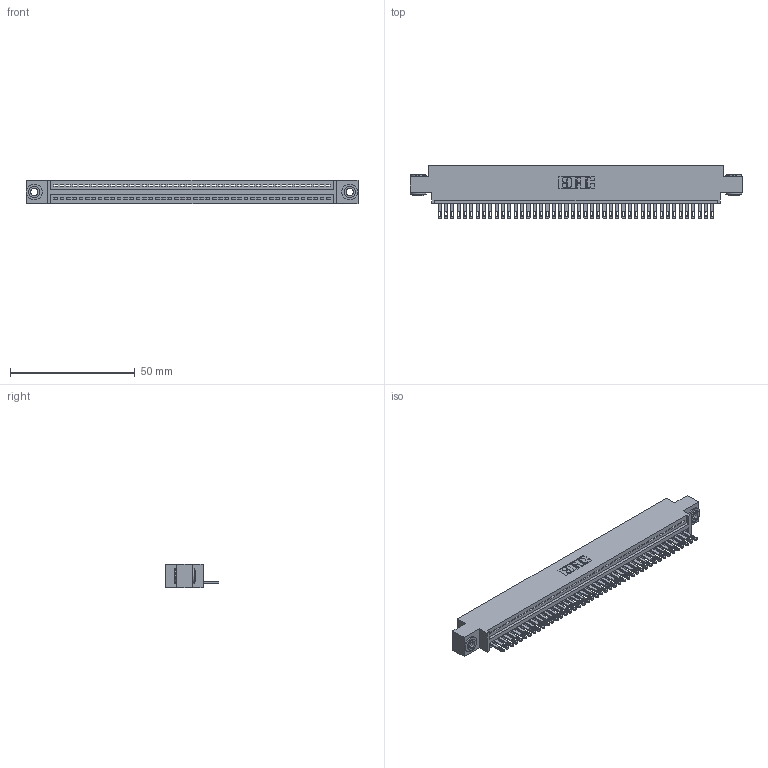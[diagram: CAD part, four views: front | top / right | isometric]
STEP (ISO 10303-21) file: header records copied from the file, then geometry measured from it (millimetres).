
FILE_DESCRIPTION (( 'STEP AP203' ), '1' );
FILE_NAME ('895-044-500-603.STEP', '2020-09-27T03:05:08', ( '' ), ( '' ), 'SwSTEP 2.0', 'SolidWorks 2020', '' );
FILE_SCHEMA (( 'CONFIG_CONTROL_DESIGN' ));
Length unit declared in the file: inch
Products named in the file (4): 345-250-002_345-250-002-102; 895-044-500-603; 845 Part_0.170 Offset - 0.156 Dia-TH; 345-292-001_345-293-100
Assembly tree (47 placements, depth 2):
  895-044-500-603
    845 Part_0.170 Offset - 0.156 Dia-TH
    345-292-001_345-293-100  x44
    345-250-002_345-250-002-102  x2
Bounding box: 132.97 x 21.51 x 9.4 mm (x, y, z)
Volume: 12579.2 mm3; surface area: 17183.6 mm2
Topology: 47 solids, 47 shells, 2544 faces, 7821 edges, 5210 vertices
Faces by surface type: plane 1590, cylinder 946, cone 8
Entity records: 33558 total; most frequent: CARTESIAN_POINT 5791, ORIENTED_EDGE 5762, DIRECTION 5087, EDGE_CURVE 2881, VECTOR 2545, LINE 2545, VERTEX_POINT 1918, AXIS2_PLACEMENT_3D 1271
